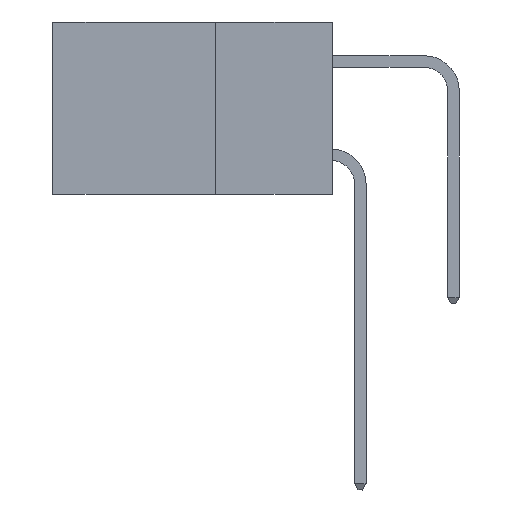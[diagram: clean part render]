
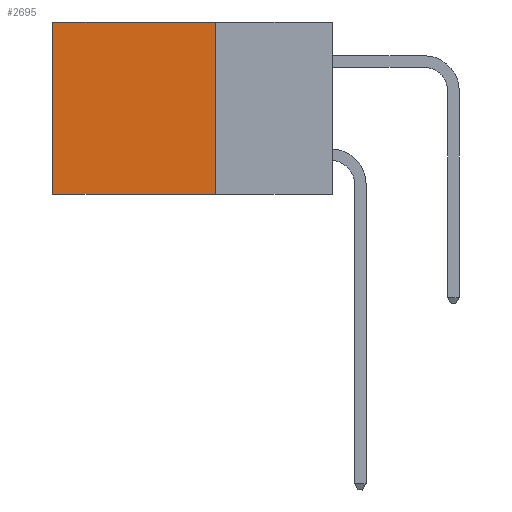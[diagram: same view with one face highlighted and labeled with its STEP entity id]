
A CAD part, left-side view. The second image highlights one B-rep face of the part: STEP entity #2695.
In plain terms, the highlighted planar face has unit normal (-1, 0, 0).
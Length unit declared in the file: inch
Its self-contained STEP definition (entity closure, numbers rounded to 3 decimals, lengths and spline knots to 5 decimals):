
#944 = CARTESIAN_POINT ( 'NONE',  ( 0.2615, 0.6, 0. ) ) ;
#1095 = EDGE_CURVE ( 'NONE', #4822, #13920, #10002, .T. ) ;
#1137 = PLANE ( 'NONE',  #16855 ) ;
#1267 = CARTESIAN_POINT ( 'NONE',  ( 0.2615, 0.25, -0.37 ) ) ;
#2695 = ADVANCED_FACE ( 'NONE', ( #15144 ), #1137, .F. ) ;
#3033 = DIRECTION ( 'NONE',  ( 1., 0., 0. ) ) ;
#3592 = VECTOR ( 'NONE', #3920, 39.37008 ) ;
#3920 = DIRECTION ( 'NONE',  ( 0., 0., -1. ) ) ;
#4041 = LINE ( 'NONE', #10855, #6166 ) ;
#4254 = DIRECTION ( 'NONE',  ( 0., 1., 0. ) ) ;
#4822 = VERTEX_POINT ( 'NONE', #5912 ) ;
#4878 = ORIENTED_EDGE ( 'NONE', *, *, #17936, .T. ) ;
#5912 = CARTESIAN_POINT ( 'NONE',  ( 0.2615, 0.25, 0. ) ) ;
#6166 = VECTOR ( 'NONE', #4254, 39.37008 ) ;
#6199 = ORIENTED_EDGE ( 'NONE', *, *, #1095, .F. ) ;
#7031 = EDGE_CURVE ( 'NONE', #13920, #16617, #9842, .T. ) ;
#7940 = ORIENTED_EDGE ( 'NONE', *, *, #7031, .F. ) ;
#9395 = LINE ( 'NONE', #12862, #3592 ) ;
#9842 = LINE ( 'NONE', #15006, #10530 ) ;
#10002 = LINE ( 'NONE', #16853, #21248 ) ;
#10530 = VECTOR ( 'NONE', #11753, 39.37008 ) ;
#10855 = CARTESIAN_POINT ( 'NONE',  ( 0.2615, 0.25, 0. ) ) ;
#11336 = DIRECTION ( 'NONE',  ( 0., 0., -1. ) ) ;
#11753 = DIRECTION ( 'NONE',  ( 0., 1., 0. ) ) ;
#12862 = CARTESIAN_POINT ( 'NONE',  ( 0.2615, 0.6, -0.37 ) ) ;
#13128 = CARTESIAN_POINT ( 'NONE',  ( 0.2615, 0.25, -0.37 ) ) ;
#13411 = CARTESIAN_POINT ( 'NONE',  ( 0.2615, 0.6, -0.37 ) ) ;
#13920 = VERTEX_POINT ( 'NONE', #1267 ) ;
#14099 = ORIENTED_EDGE ( 'NONE', *, *, #15131, .T. ) ;
#15006 = CARTESIAN_POINT ( 'NONE',  ( 0.2615, 0.25, -0.37 ) ) ;
#15131 = EDGE_CURVE ( 'NONE', #16961, #16617, #9395, .T. ) ;
#15144 = FACE_OUTER_BOUND ( 'NONE', #15817, .T. ) ;
#15817 = EDGE_LOOP ( 'NONE', ( #14099, #7940, #6199, #4878 ) ) ;
#16617 = VERTEX_POINT ( 'NONE', #13411 ) ;
#16853 = CARTESIAN_POINT ( 'NONE',  ( 0.2615, 0.25, -0.37 ) ) ;
#16855 = AXIS2_PLACEMENT_3D ( 'NONE', #13128, #3033, #11336 ) ;
#16961 = VERTEX_POINT ( 'NONE', #944 ) ;
#17936 = EDGE_CURVE ( 'NONE', #4822, #16961, #4041, .T. ) ;
#19778 = DIRECTION ( 'NONE',  ( 0., 0., -1. ) ) ;
#21248 = VECTOR ( 'NONE', #19778, 39.37008 ) ;
